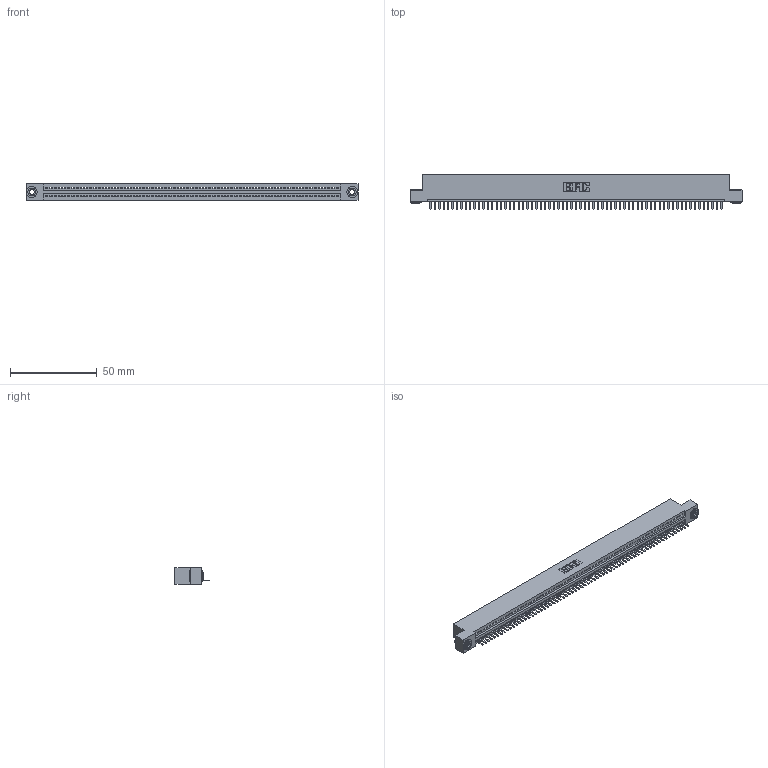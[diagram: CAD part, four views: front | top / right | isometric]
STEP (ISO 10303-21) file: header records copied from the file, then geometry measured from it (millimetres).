
FILE_DESCRIPTION (( 'STEP AP203' ), '1' );
FILE_NAME ('395-067-520-103.STEP', '2018-11-25T07:33:04', ( '' ), ( '' ), 'SwSTEP 2.0', 'SolidWorks 2016', '' );
FILE_SCHEMA (( 'CONFIG_CONTROL_DESIGN' ));
Length unit declared in the file: inch
Products named in the file (4): 345-250-002_345-250-002-102; 395-067-520-103; 345-292-001_345-293-120; 345 Part_Flush Mounting Lugs - 0.156 Dia-TH
Assembly tree (70 placements, depth 2):
  395-067-520-103
    345 Part_Flush Mounting Lugs - 0.156 Dia-TH
    345-292-001_345-293-120  x67
    345-250-002_345-250-002-102  x2
Bounding box: 191.39 x 19.68 x 9.4 mm (x, y, z)
Volume: 18209.8 mm3; surface area: 24122.9 mm2
Topology: 70 solids, 70 shells, 4318 faces, 12745 edges, 8314 vertices
Faces by surface type: plane 2904, cylinder 1406, cone 8
Entity records: 47824 total; most frequent: CARTESIAN_POINT 8272, ORIENTED_EDGE 8254, DIRECTION 7207, EDGE_CURVE 4127, VECTOR 3699, LINE 3699, VERTEX_POINT 2746, AXIS2_PLACEMENT_3D 1754
